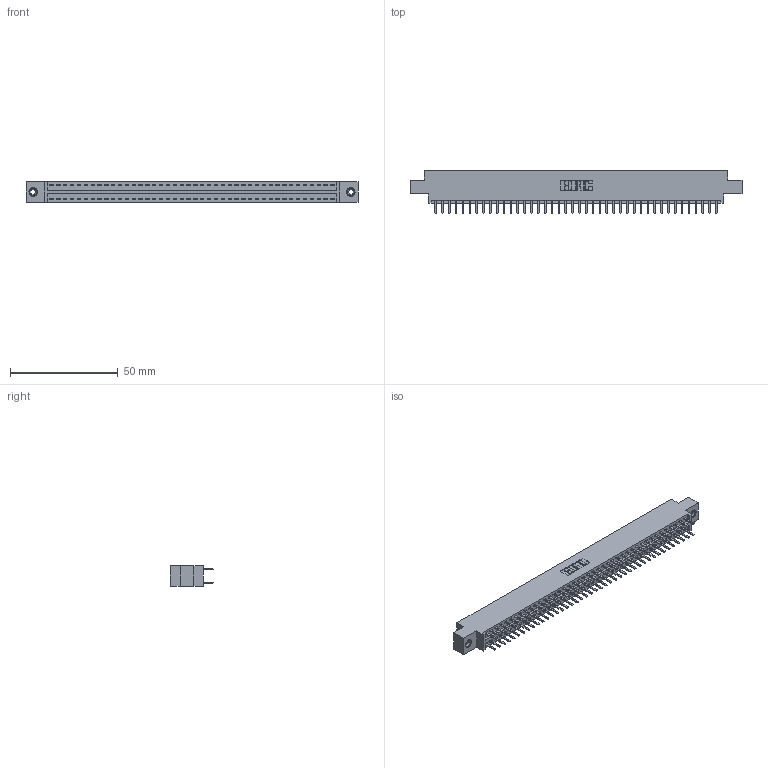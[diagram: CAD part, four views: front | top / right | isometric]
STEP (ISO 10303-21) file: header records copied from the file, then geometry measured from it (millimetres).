
FILE_DESCRIPTION (( 'STEP AP203' ), '1' );
FILE_NAME ('396-084-520-808.STEP', '2019-11-02T14:15:40', ( '' ), ( '' ), 'SwSTEP 2.0', 'SolidWorks 2016', '' );
FILE_SCHEMA (( 'CONFIG_CONTROL_DESIGN' ));
Length unit declared in the file: inch
Products named in the file (4): 346 Part_0.170 Offset - 0.156 Dia-TI; 345-292-001_345-293-120; 345-250-001_345-250-003-102; 396-084-520-808
Assembly tree (87 placements, depth 2):
  396-084-520-808
    346 Part_0.170 Offset - 0.156 Dia-TI
    345-292-001_345-293-120  x84
    345-250-001_345-250-003-102  x2
Bounding box: 153.92 x 20.02 x 9.4 mm (x, y, z)
Volume: 14811.4 mm3; surface area: 20472.5 mm2
Topology: 87 solids, 87 shells, 4890 faces, 14169 edges, 9214 vertices
Faces by surface type: plane 3220, cylinder 1654, cone 12, torus 4
Entity records: 28842 total; most frequent: CARTESIAN_POINT 4751, ORIENTED_EDGE 4666, DIRECTION 4251, EDGE_CURVE 2333, VECTOR 2009, LINE 2009, VERTEX_POINT 1548, AXIS2_PLACEMENT_3D 1121
